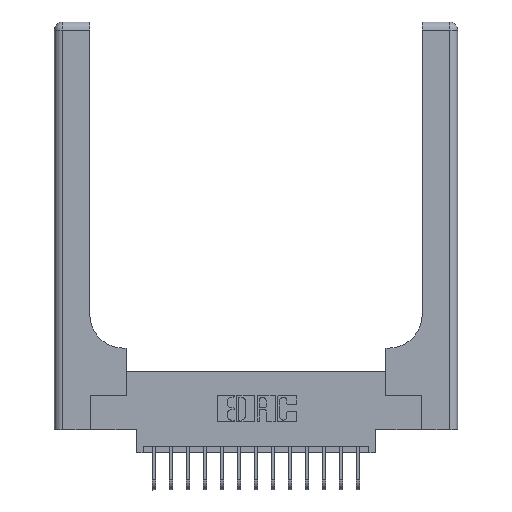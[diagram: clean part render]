
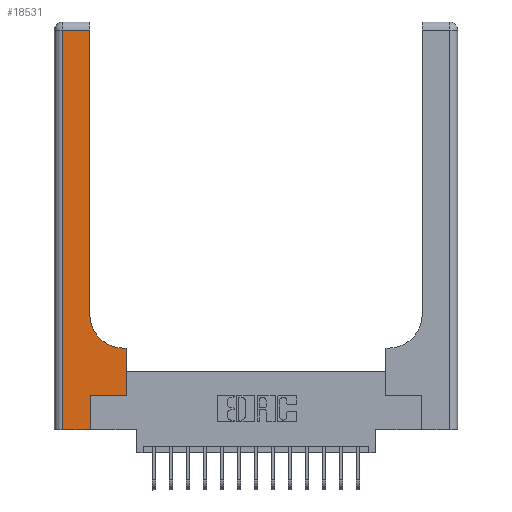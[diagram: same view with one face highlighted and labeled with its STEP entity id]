
A CAD part, top view. The second image highlights one B-rep face of the part: STEP entity #18531.
In plain terms, the highlighted planar face has unit normal (0, 0, 1).
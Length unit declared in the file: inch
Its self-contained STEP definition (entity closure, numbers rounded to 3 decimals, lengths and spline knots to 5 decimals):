
#262 = LINE ( 'NONE', #1585, #14930 ) ;
#315 = ORIENTED_EDGE ( 'NONE', *, *, #1339, .T. ) ;
#604 = CARTESIAN_POINT ( 'NONE',  ( 0.51, 0.6, 0.37 ) ) ;
#736 = AXIS2_PLACEMENT_3D ( 'NONE', #8795, #14011, #9511 ) ;
#971 = DIRECTION ( 'NONE',  ( -1., 0., 0. ) ) ;
#1085 = VECTOR ( 'NONE', #15165, 39.37008 ) ;
#1339 = EDGE_CURVE ( 'NONE', #13574, #2436, #3377, .T. ) ;
#1522 = CARTESIAN_POINT ( 'NONE',  ( 0.265, 0., 0.37 ) ) ;
#1585 = CARTESIAN_POINT ( 'NONE',  ( 0.26, 3., 0.37 ) ) ;
#1592 = EDGE_CURVE ( 'NONE', #10415, #12259, #5724, .T. ) ;
#1990 = AXIS2_PLACEMENT_3D ( 'NONE', #15448, #7960, #18484 ) ;
#2436 = VERTEX_POINT ( 'NONE', #604 ) ;
#2465 = CARTESIAN_POINT ( 'NONE',  ( 0.06, 0., 0.37 ) ) ;
#2679 = EDGE_CURVE ( 'NONE', #3111, #13042, #16279, .T. ) ;
#3111 = VERTEX_POINT ( 'NONE', #12848 ) ;
#3195 = DIRECTION ( 'NONE',  ( 0., 1., 0. ) ) ;
#3342 = EDGE_LOOP ( 'NONE', ( #5022, #18221, #11490, #6771, #9588, #12269, #8452, #315, #15709 ) ) ;
#3377 = LINE ( 'NONE', #5384, #6453 ) ;
#4108 = CARTESIAN_POINT ( 'NONE',  ( 0.265, 0., 0.37 ) ) ;
#4155 = VERTEX_POINT ( 'NONE', #17316 ) ;
#4753 = PLANE ( 'NONE',  #1990 ) ;
#4906 = CARTESIAN_POINT ( 'NONE',  ( 0.06, 3., 0.37 ) ) ;
#5022 = ORIENTED_EDGE ( 'NONE', *, *, #5512, .T. ) ;
#5384 = CARTESIAN_POINT ( 'NONE',  ( 0.26, 0.6, 0.37 ) ) ;
#5512 = EDGE_CURVE ( 'NONE', #4155, #3111, #262, .T. ) ;
#5621 = DIRECTION ( 'NONE',  ( 0., 1., 0. ) ) ;
#5724 = LINE ( 'NONE', #15157, #9763 ) ;
#6175 = VERTEX_POINT ( 'NONE', #12694 ) ;
#6438 = CARTESIAN_POINT ( 'NONE',  ( 0.528, 0.25, 0.37 ) ) ;
#6453 = VECTOR ( 'NONE', #971, 39.37008 ) ;
#6591 = VECTOR ( 'NONE', #5621, 39.37008 ) ;
#6629 = EDGE_CURVE ( 'NONE', #2436, #4155, #11614, .T. ) ;
#6630 = LINE ( 'NONE', #4906, #12993 ) ;
#6771 = ORIENTED_EDGE ( 'NONE', *, *, #1592, .T. ) ;
#6795 = CARTESIAN_POINT ( 'NONE',  ( 0., 2.94, 0.37 ) ) ;
#7247 = LINE ( 'NONE', #13629, #1085 ) ;
#7428 = EDGE_CURVE ( 'NONE', #12259, #6175, #17896, .T. ) ;
#7672 = DIRECTION ( 'NONE',  ( 0., 1., 0. ) ) ;
#7684 = CARTESIAN_POINT ( 'NONE',  ( 0.528, 0.6, 0.37 ) ) ;
#7960 = DIRECTION ( 'NONE',  ( 0., 0., -1. ) ) ;
#8132 = DIRECTION ( 'NONE',  ( 0., -1., 0. ) ) ;
#8452 = ORIENTED_EDGE ( 'NONE', *, *, #11325, .T. ) ;
#8795 = CARTESIAN_POINT ( 'NONE',  ( 0.51, 0.85, 0.37 ) ) ;
#9170 = EDGE_CURVE ( 'NONE', #6175, #9330, #7247, .T. ) ;
#9330 = VERTEX_POINT ( 'NONE', #17233 ) ;
#9425 = CARTESIAN_POINT ( 'NONE',  ( 0.06, 2.94, 0.37 ) ) ;
#9511 = DIRECTION ( 'NONE',  ( 1., 0., 0. ) ) ;
#9588 = ORIENTED_EDGE ( 'NONE', *, *, #7428, .T. ) ;
#9763 = VECTOR ( 'NONE', #10761, 39.37008 ) ;
#10415 = VERTEX_POINT ( 'NONE', #2465 ) ;
#10761 = DIRECTION ( 'NONE',  ( 1., 0., 0. ) ) ;
#11165 = VECTOR ( 'NONE', #3195, 39.37008 ) ;
#11320 = VECTOR ( 'NONE', #17337, 39.37008 ) ;
#11325 = EDGE_CURVE ( 'NONE', #9330, #13574, #16358, .T. ) ;
#11490 = ORIENTED_EDGE ( 'NONE', *, *, #17224, .T. ) ;
#11614 = CIRCLE ( 'NONE', #736, 0.25 ) ;
#12259 = VERTEX_POINT ( 'NONE', #1522 ) ;
#12269 = ORIENTED_EDGE ( 'NONE', *, *, #9170, .T. ) ;
#12694 = CARTESIAN_POINT ( 'NONE',  ( 0.265, 0.25, 0.37 ) ) ;
#12848 = CARTESIAN_POINT ( 'NONE',  ( 0.26, 2.94, 0.37 ) ) ;
#12985 = FACE_OUTER_BOUND ( 'NONE', #3342, .T. ) ;
#12993 = VECTOR ( 'NONE', #8132, 39.37008 ) ;
#13042 = VERTEX_POINT ( 'NONE', #9425 ) ;
#13574 = VERTEX_POINT ( 'NONE', #7684 ) ;
#13629 = CARTESIAN_POINT ( 'NONE',  ( 0.265, 0.25, 0.37 ) ) ;
#14011 = DIRECTION ( 'NONE',  ( 0., 0., -1. ) ) ;
#14930 = VECTOR ( 'NONE', #7672, 39.37008 ) ;
#15157 = CARTESIAN_POINT ( 'NONE',  ( 0., 0., 0.37 ) ) ;
#15165 = DIRECTION ( 'NONE',  ( 1., 0., 0. ) ) ;
#15448 = CARTESIAN_POINT ( 'NONE',  ( 0., 3., 0.37 ) ) ;
#15709 = ORIENTED_EDGE ( 'NONE', *, *, #6629, .T. ) ;
#16279 = LINE ( 'NONE', #6795, #11320 ) ;
#16358 = LINE ( 'NONE', #6438, #11165 ) ;
#17224 = EDGE_CURVE ( 'NONE', #13042, #10415, #6630, .T. ) ;
#17233 = CARTESIAN_POINT ( 'NONE',  ( 0.528, 0.25, 0.37 ) ) ;
#17316 = CARTESIAN_POINT ( 'NONE',  ( 0.26, 0.85, 0.37 ) ) ;
#17337 = DIRECTION ( 'NONE',  ( -1., 0., 0. ) ) ;
#17896 = LINE ( 'NONE', #4108, #6591 ) ;
#18221 = ORIENTED_EDGE ( 'NONE', *, *, #2679, .T. ) ;
#18484 = DIRECTION ( 'NONE',  ( -1., 0., 0. ) ) ;
#18531 = ADVANCED_FACE ( 'NONE', ( #12985 ), #4753, .F. ) ;
